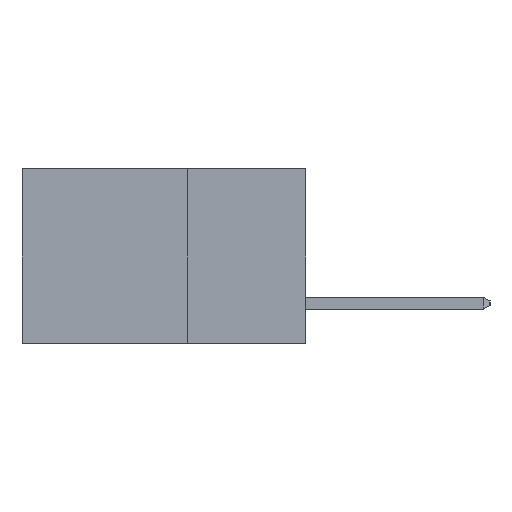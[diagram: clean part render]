
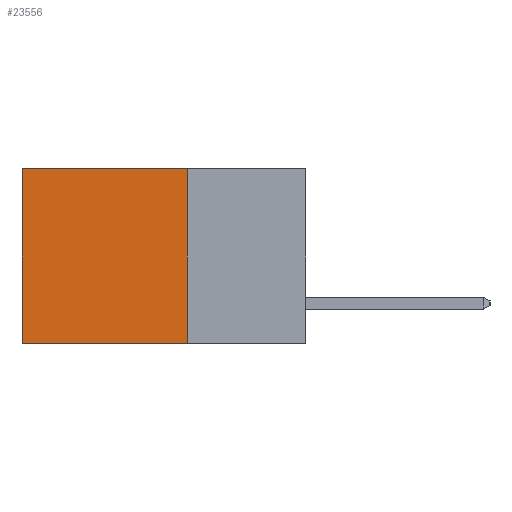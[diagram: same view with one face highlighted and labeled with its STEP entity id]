
A CAD part, left-side view. The second image highlights one B-rep face of the part: STEP entity #23556.
In plain terms, the highlighted planar face has unit normal (-1, 0, 0).
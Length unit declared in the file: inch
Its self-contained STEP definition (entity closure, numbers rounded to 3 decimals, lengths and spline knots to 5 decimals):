
#208 = VECTOR ( 'NONE', #18966, 39.37008 ) ;
#238 = CARTESIAN_POINT ( 'NONE',  ( 0.2615, 0.25, -0.37 ) ) ;
#457 = DIRECTION ( 'NONE',  ( 0., 0., -1. ) ) ;
#486 = VECTOR ( 'NONE', #457, 39.37008 ) ;
#825 = LINE ( 'NONE', #3545, #20668 ) ;
#1200 = CARTESIAN_POINT ( 'NONE',  ( 0.2615, 0.6, -0.37 ) ) ;
#2255 = DIRECTION ( 'NONE',  ( 1., 0., 0. ) ) ;
#2656 = ORIENTED_EDGE ( 'NONE', *, *, #19405, .T. ) ;
#2910 = VERTEX_POINT ( 'NONE', #12828 ) ;
#2951 = EDGE_LOOP ( 'NONE', ( #24516, #15636, #12707, #2656 ) ) ;
#3545 = CARTESIAN_POINT ( 'NONE',  ( 0.2615, 0.25, 0. ) ) ;
#5567 = DIRECTION ( 'NONE',  ( 0., 1., 0. ) ) ;
#9643 = EDGE_CURVE ( 'NONE', #20414, #18783, #20334, .T. ) ;
#9936 = DIRECTION ( 'NONE',  ( 0., 0., -1. ) ) ;
#9939 = CARTESIAN_POINT ( 'NONE',  ( 0.2615, 0.25, -0.37 ) ) ;
#12707 = ORIENTED_EDGE ( 'NONE', *, *, #15120, .F. ) ;
#12828 = CARTESIAN_POINT ( 'NONE',  ( 0.2615, 0.25, -0.37 ) ) ;
#14190 = LINE ( 'NONE', #9939, #19168 ) ;
#14482 = EDGE_CURVE ( 'NONE', #2910, #18783, #16921, .T. ) ;
#14980 = AXIS2_PLACEMENT_3D ( 'NONE', #238, #2255, #15791 ) ;
#15120 = EDGE_CURVE ( 'NONE', #18234, #2910, #14190, .T. ) ;
#15636 = ORIENTED_EDGE ( 'NONE', *, *, #14482, .F. ) ;
#15791 = DIRECTION ( 'NONE',  ( 0., 0., -1. ) ) ;
#16921 = LINE ( 'NONE', #19112, #208 ) ;
#17909 = FACE_OUTER_BOUND ( 'NONE', #2951, .T. ) ;
#18234 = VERTEX_POINT ( 'NONE', #23463 ) ;
#18783 = VERTEX_POINT ( 'NONE', #21412 ) ;
#18966 = DIRECTION ( 'NONE',  ( 0., 1., 0. ) ) ;
#19112 = CARTESIAN_POINT ( 'NONE',  ( 0.2615, 0.25, -0.37 ) ) ;
#19168 = VECTOR ( 'NONE', #9936, 39.37008 ) ;
#19405 = EDGE_CURVE ( 'NONE', #18234, #20414, #825, .T. ) ;
#19957 = CARTESIAN_POINT ( 'NONE',  ( 0.2615, 0.6, 0. ) ) ;
#20334 = LINE ( 'NONE', #1200, #486 ) ;
#20414 = VERTEX_POINT ( 'NONE', #19957 ) ;
#20668 = VECTOR ( 'NONE', #5567, 39.37008 ) ;
#21412 = CARTESIAN_POINT ( 'NONE',  ( 0.2615, 0.6, -0.37 ) ) ;
#23201 = PLANE ( 'NONE',  #14980 ) ;
#23463 = CARTESIAN_POINT ( 'NONE',  ( 0.2615, 0.25, 0. ) ) ;
#23556 = ADVANCED_FACE ( 'NONE', ( #17909 ), #23201, .F. ) ;
#24516 = ORIENTED_EDGE ( 'NONE', *, *, #9643, .T. ) ;
